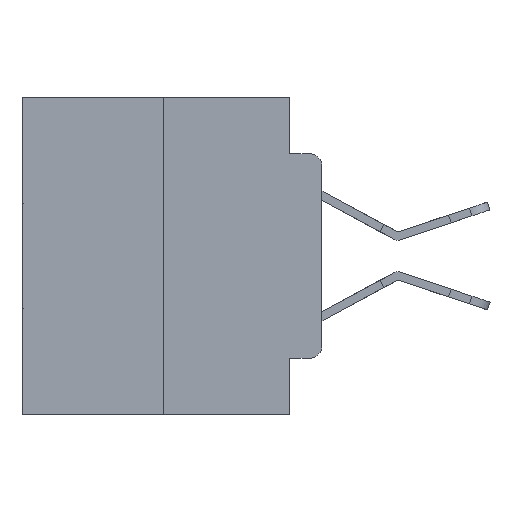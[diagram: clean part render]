
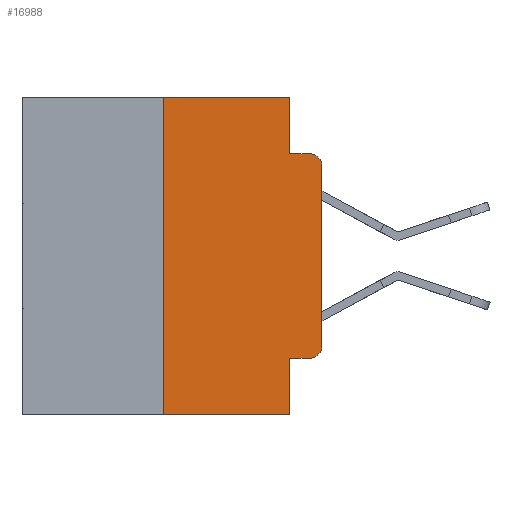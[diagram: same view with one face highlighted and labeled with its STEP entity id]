
A CAD part, left-side view. The second image highlights one B-rep face of the part: STEP entity #16988.
In plain terms, the highlighted planar face has unit normal (-1, 0, 0).
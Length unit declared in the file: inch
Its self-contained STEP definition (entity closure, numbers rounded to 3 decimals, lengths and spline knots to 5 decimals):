
#506 = EDGE_CURVE ( 'NONE', #6454, #25349, #14115, .T. ) ;
#533 = LINE ( 'NONE', #15705, #24074 ) ;
#1254 = LINE ( 'NONE', #28633, #17197 ) ;
#1283 = ORIENTED_EDGE ( 'NONE', *, *, #4231, .T. ) ;
#1669 = VERTEX_POINT ( 'NONE', #13682 ) ;
#1697 = EDGE_CURVE ( 'NONE', #1669, #21924, #533, .T. ) ;
#1854 = VECTOR ( 'NONE', #19649, 39.37008 ) ;
#2110 = EDGE_CURVE ( 'NONE', #24864, #3259, #17135, .T. ) ;
#2238 = CARTESIAN_POINT ( 'NONE',  ( 0., 0.051, -0.5 ) ) ;
#2530 = PLANE ( 'NONE',  #15809 ) ;
#2534 = LINE ( 'NONE', #8467, #3945 ) ;
#2615 = DIRECTION ( 'NONE',  ( 0., -1., 0. ) ) ;
#2752 = EDGE_CURVE ( 'NONE', #3259, #12354, #16088, .T. ) ;
#3259 = VERTEX_POINT ( 'NONE', #21495 ) ;
#3360 = EDGE_CURVE ( 'NONE', #24864, #21924, #2534, .T. ) ;
#3945 = VECTOR ( 'NONE', #23926, 39.37008 ) ;
#4128 = CARTESIAN_POINT ( 'NONE',  ( 0., 0.02, -0.1085 ) ) ;
#4231 = EDGE_CURVE ( 'NONE', #27877, #17969, #19317, .T. ) ;
#4265 = DIRECTION ( 'NONE',  ( 0., -1., 0. ) ) ;
#4472 = ORIENTED_EDGE ( 'NONE', *, *, #3360, .F. ) ;
#4946 = VECTOR ( 'NONE', #15904, 39.37008 ) ;
#5401 = CARTESIAN_POINT ( 'NONE',  ( 0., 0., -0.3915 ) ) ;
#5564 = CARTESIAN_POINT ( 'NONE',  ( 0., 0., -0.1085 ) ) ;
#6147 = CARTESIAN_POINT ( 'NONE',  ( 0., 0.02, -0.3915 ) ) ;
#6454 = VERTEX_POINT ( 'NONE', #21226 ) ;
#6969 = ORIENTED_EDGE ( 'NONE', *, *, #506, .F. ) ;
#7145 = AXIS2_PLACEMENT_3D ( 'NONE', #6147, #13115, #12823 ) ;
#7633 = DIRECTION ( 'NONE',  ( 0., 0., -1. ) ) ;
#8467 = CARTESIAN_POINT ( 'NONE',  ( 0., 0.051, 0. ) ) ;
#8481 = CARTESIAN_POINT ( 'NONE',  ( 0., 0.25, 0. ) ) ;
#9467 = VERTEX_POINT ( 'NONE', #9606 ) ;
#9549 = EDGE_CURVE ( 'NONE', #25349, #9467, #15251, .T. ) ;
#9606 = CARTESIAN_POINT ( 'NONE',  ( 0., 0.051, -0.0885 ) ) ;
#10926 = DIRECTION ( 'NONE',  ( 0., 0., 1. ) ) ;
#11445 = CARTESIAN_POINT ( 'NONE',  ( 0., 0.051, -0.0885 ) ) ;
#12226 = LINE ( 'NONE', #11445, #4946 ) ;
#12354 = VERTEX_POINT ( 'NONE', #5401 ) ;
#12548 = CARTESIAN_POINT ( 'NONE',  ( 0., 0.02, -0.0885 ) ) ;
#12823 = DIRECTION ( 'NONE',  ( 0., 0., -1. ) ) ;
#13115 = DIRECTION ( 'NONE',  ( -1., 0., 0. ) ) ;
#13682 = CARTESIAN_POINT ( 'NONE',  ( 0., 0.25, -0.5 ) ) ;
#13789 = VECTOR ( 'NONE', #4265, 39.37008 ) ;
#13980 = CARTESIAN_POINT ( 'NONE',  ( 0., 0.473, 0. ) ) ;
#14115 = LINE ( 'NONE', #19743, #13789 ) ;
#14981 = DIRECTION ( 'NONE',  ( 0., 0., -1. ) ) ;
#15251 = LINE ( 'NONE', #27749, #18353 ) ;
#15705 = CARTESIAN_POINT ( 'NONE',  ( 0., 0.473, -0.5 ) ) ;
#15809 = AXIS2_PLACEMENT_3D ( 'NONE', #13980, #22461, #22749 ) ;
#15904 = DIRECTION ( 'NONE',  ( 0., -1., 0. ) ) ;
#16088 = CIRCLE ( 'NONE', #7145, 0.02 ) ;
#16700 = EDGE_CURVE ( 'NONE', #1669, #6454, #23343, .T. ) ;
#16988 = ADVANCED_FACE ( 'NONE', ( #19611 ), #2530, .F. ) ;
#17135 = LINE ( 'NONE', #17417, #1854 ) ;
#17197 = VECTOR ( 'NONE', #10926, 39.37008 ) ;
#17366 = DIRECTION ( 'NONE',  ( 0., 0., 1. ) ) ;
#17417 = CARTESIAN_POINT ( 'NONE',  ( 0., 0.051, -0.4115 ) ) ;
#17969 = VERTEX_POINT ( 'NONE', #12548 ) ;
#18203 = ORIENTED_EDGE ( 'NONE', *, *, #16700, .F. ) ;
#18353 = VECTOR ( 'NONE', #7633, 39.37008 ) ;
#18550 = ORIENTED_EDGE ( 'NONE', *, *, #28356, .F. ) ;
#19240 = VECTOR ( 'NONE', #17366, 39.37008 ) ;
#19317 = CIRCLE ( 'NONE', #21079, 0.02 ) ;
#19611 = FACE_OUTER_BOUND ( 'NONE', #28353, .T. ) ;
#19649 = DIRECTION ( 'NONE',  ( 0., -1., 0. ) ) ;
#19743 = CARTESIAN_POINT ( 'NONE',  ( 0., 0.473, 0. ) ) ;
#21079 = AXIS2_PLACEMENT_3D ( 'NONE', #4128, #28026, #14981 ) ;
#21112 = ORIENTED_EDGE ( 'NONE', *, *, #2110, .T. ) ;
#21226 = CARTESIAN_POINT ( 'NONE',  ( 0., 0.25, 0. ) ) ;
#21495 = CARTESIAN_POINT ( 'NONE',  ( 0., 0.02, -0.4115 ) ) ;
#21924 = VERTEX_POINT ( 'NONE', #2238 ) ;
#22461 = DIRECTION ( 'NONE',  ( 1., 0., 0. ) ) ;
#22749 = DIRECTION ( 'NONE',  ( 0., 0., -1. ) ) ;
#22861 = ORIENTED_EDGE ( 'NONE', *, *, #1697, .T. ) ;
#23070 = CARTESIAN_POINT ( 'NONE',  ( 0., 0.051, -0.4115 ) ) ;
#23343 = LINE ( 'NONE', #8481, #19240 ) ;
#23926 = DIRECTION ( 'NONE',  ( 0., 0., -1. ) ) ;
#23988 = ORIENTED_EDGE ( 'NONE', *, *, #25666, .T. ) ;
#24074 = VECTOR ( 'NONE', #2615, 39.37008 ) ;
#24864 = VERTEX_POINT ( 'NONE', #23070 ) ;
#25349 = VERTEX_POINT ( 'NONE', #25618 ) ;
#25618 = CARTESIAN_POINT ( 'NONE',  ( 0., 0.051, 0. ) ) ;
#25666 = EDGE_CURVE ( 'NONE', #12354, #27877, #1254, .T. ) ;
#25801 = ORIENTED_EDGE ( 'NONE', *, *, #2752, .T. ) ;
#27696 = ORIENTED_EDGE ( 'NONE', *, *, #9549, .F. ) ;
#27749 = CARTESIAN_POINT ( 'NONE',  ( 0., 0.051, 0. ) ) ;
#27877 = VERTEX_POINT ( 'NONE', #5564 ) ;
#28026 = DIRECTION ( 'NONE',  ( -1., 0., 0. ) ) ;
#28353 = EDGE_LOOP ( 'NONE', ( #23988, #1283, #18550, #27696, #6969, #18203, #22861, #4472, #21112, #25801 ) ) ;
#28356 = EDGE_CURVE ( 'NONE', #9467, #17969, #12226, .T. ) ;
#28633 = CARTESIAN_POINT ( 'NONE',  ( 0., 0., 0. ) ) ;
